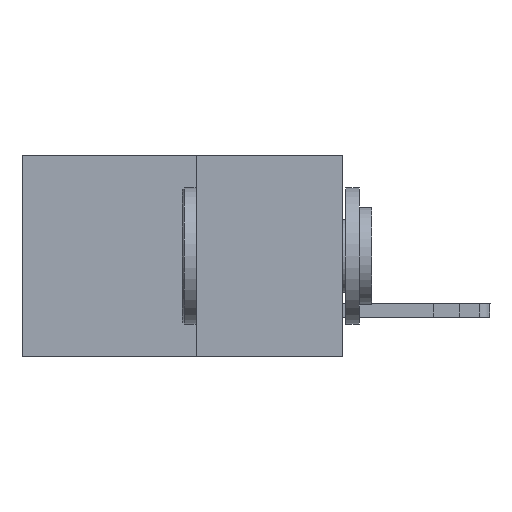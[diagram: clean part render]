
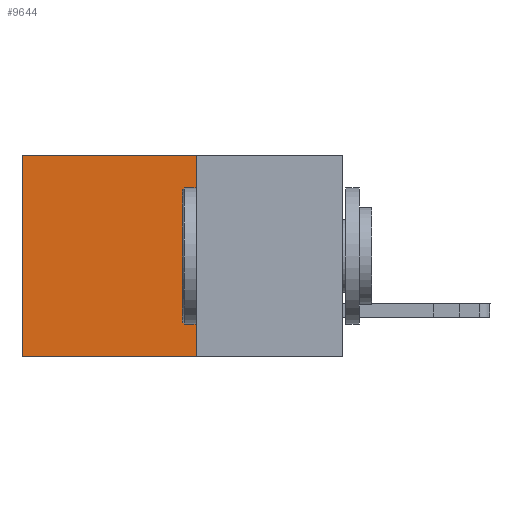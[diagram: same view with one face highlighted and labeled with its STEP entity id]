
A CAD part, left-side view. The second image highlights one B-rep face of the part: STEP entity #9644.
In plain terms, the highlighted planar face has unit normal (-1, 0, 0).
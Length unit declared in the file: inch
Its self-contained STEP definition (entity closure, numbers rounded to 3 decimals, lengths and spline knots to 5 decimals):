
#455 = ORIENTED_EDGE ( 'NONE', *, *, #3363, .F. ) ;
#959 = ORIENTED_EDGE ( 'NONE', *, *, #3623, .T. ) ;
#1427 = DIRECTION ( 'NONE',  ( 1., 0., 0. ) ) ;
#1577 = VERTEX_POINT ( 'NONE', #10419 ) ;
#1899 = VERTEX_POINT ( 'NONE', #2573 ) ;
#1932 = EDGE_CURVE ( 'NONE', #1577, #16139, #11774, .T. ) ;
#2517 = VECTOR ( 'NONE', #12013, 39.37008 ) ;
#2573 = CARTESIAN_POINT ( 'NONE',  ( 0.277, 0.27, -0.37 ) ) ;
#2953 = VECTOR ( 'NONE', #18593, 39.37008 ) ;
#3363 = EDGE_CURVE ( 'NONE', #1899, #16139, #12448, .T. ) ;
#3623 = EDGE_CURVE ( 'NONE', #12184, #1577, #8895, .T. ) ;
#3745 = CARTESIAN_POINT ( 'NONE',  ( 0.277, 0.59, -0.37 ) ) ;
#5369 = EDGE_LOOP ( 'NONE', ( #12999, #455, #9183, #959 ) ) ;
#5626 = LINE ( 'NONE', #5689, #7960 ) ;
#5689 = CARTESIAN_POINT ( 'NONE',  ( 0.277, 0.27, -0.37 ) ) ;
#7960 = VECTOR ( 'NONE', #12266, 39.37008 ) ;
#8197 = CARTESIAN_POINT ( 'NONE',  ( 0.277, 0.59, -0.37 ) ) ;
#8895 = LINE ( 'NONE', #16998, #2953 ) ;
#9183 = ORIENTED_EDGE ( 'NONE', *, *, #13659, .F. ) ;
#9644 = ADVANCED_FACE ( 'NONE', ( #14520 ), #21162, .F. ) ;
#10125 = AXIS2_PLACEMENT_3D ( 'NONE', #11258, #1427, #12891 ) ;
#10419 = CARTESIAN_POINT ( 'NONE',  ( 0.277, 0.59, 0. ) ) ;
#11258 = CARTESIAN_POINT ( 'NONE',  ( 0.277, 0.27, -0.37 ) ) ;
#11774 = LINE ( 'NONE', #3745, #2517 ) ;
#12013 = DIRECTION ( 'NONE',  ( 0., 0., -1. ) ) ;
#12184 = VERTEX_POINT ( 'NONE', #16150 ) ;
#12266 = DIRECTION ( 'NONE',  ( 0., 0., -1. ) ) ;
#12448 = LINE ( 'NONE', #18542, #16377 ) ;
#12891 = DIRECTION ( 'NONE',  ( 0., 0., -1. ) ) ;
#12999 = ORIENTED_EDGE ( 'NONE', *, *, #1932, .T. ) ;
#13659 = EDGE_CURVE ( 'NONE', #12184, #1899, #5626, .T. ) ;
#14520 = FACE_OUTER_BOUND ( 'NONE', #5369, .T. ) ;
#16139 = VERTEX_POINT ( 'NONE', #8197 ) ;
#16150 = CARTESIAN_POINT ( 'NONE',  ( 0.277, 0.27, 0. ) ) ;
#16377 = VECTOR ( 'NONE', #18634, 39.37008 ) ;
#16998 = CARTESIAN_POINT ( 'NONE',  ( 0.277, 0.27, 0. ) ) ;
#18542 = CARTESIAN_POINT ( 'NONE',  ( 0.277, 0.27, -0.37 ) ) ;
#18593 = DIRECTION ( 'NONE',  ( 0., 1., 0. ) ) ;
#18634 = DIRECTION ( 'NONE',  ( 0., 1., 0. ) ) ;
#21162 = PLANE ( 'NONE',  #10125 ) ;
